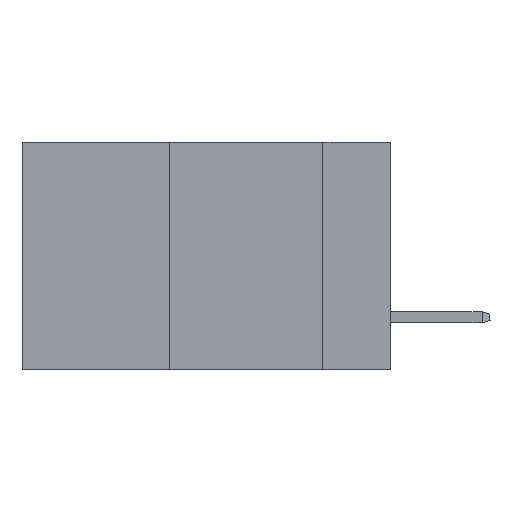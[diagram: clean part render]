
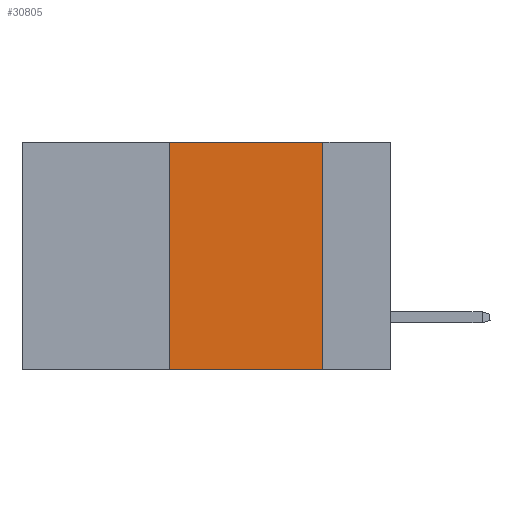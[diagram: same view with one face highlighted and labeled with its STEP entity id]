
A CAD part, left-side view. The second image highlights one B-rep face of the part: STEP entity #30805.
In plain terms, the highlighted planar face has unit normal (-1, 0, 0).
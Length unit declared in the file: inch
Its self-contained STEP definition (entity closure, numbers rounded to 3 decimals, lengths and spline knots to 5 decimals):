
#793 = VERTEX_POINT ( 'NONE', #25462 ) ;
#969 = DIRECTION ( 'NONE',  ( 0., -1., 0. ) ) ;
#1137 = VECTOR ( 'NONE', #1248, 39.37008 ) ;
#1248 = DIRECTION ( 'NONE',  ( 0., -1., 0. ) ) ;
#3968 = VECTOR ( 'NONE', #23589, 39.37008 ) ;
#4035 = CARTESIAN_POINT ( 'NONE',  ( 0., 0.11, 0. ) ) ;
#8801 = EDGE_LOOP ( 'NONE', ( #17705, #30696, #17278, #35074 ) ) ;
#9287 = VERTEX_POINT ( 'NONE', #24749 ) ;
#9835 = CARTESIAN_POINT ( 'NONE',  ( 0., 0.36, 0. ) ) ;
#10026 = VECTOR ( 'NONE', #33247, 39.37008 ) ;
#10438 = LINE ( 'NONE', #22351, #1137 ) ;
#13290 = CARTESIAN_POINT ( 'NONE',  ( 0., 0.6, 0. ) ) ;
#13874 = AXIS2_PLACEMENT_3D ( 'NONE', #13290, #28423, #22605 ) ;
#14196 = EDGE_CURVE ( 'NONE', #793, #27697, #25897, .T. ) ;
#14399 = EDGE_CURVE ( 'NONE', #27697, #33178, #10438, .T. ) ;
#17278 = ORIENTED_EDGE ( 'NONE', *, *, #14196, .F. ) ;
#17705 = ORIENTED_EDGE ( 'NONE', *, *, #26358, .F. ) ;
#19092 = VECTOR ( 'NONE', #969, 39.37008 ) ;
#22351 = CARTESIAN_POINT ( 'NONE',  ( 0., 0.6, 0. ) ) ;
#22605 = DIRECTION ( 'NONE',  ( 0., 0., -1. ) ) ;
#23589 = DIRECTION ( 'NONE',  ( 0., 0., -1. ) ) ;
#24749 = CARTESIAN_POINT ( 'NONE',  ( 0., 0.11, -0.37 ) ) ;
#25462 = CARTESIAN_POINT ( 'NONE',  ( 0., 0.36, -0.37 ) ) ;
#25628 = CARTESIAN_POINT ( 'NONE',  ( 0., 0.36, 0. ) ) ;
#25897 = LINE ( 'NONE', #9835, #10026 ) ;
#26358 = EDGE_CURVE ( 'NONE', #33178, #9287, #38029, .T. ) ;
#26664 = CARTESIAN_POINT ( 'NONE',  ( 0., 0.11, 0. ) ) ;
#27017 = LINE ( 'NONE', #31013, #19092 ) ;
#27697 = VERTEX_POINT ( 'NONE', #25628 ) ;
#28423 = DIRECTION ( 'NONE',  ( 1., 0., 0. ) ) ;
#30696 = ORIENTED_EDGE ( 'NONE', *, *, #14399, .F. ) ;
#30805 = ADVANCED_FACE ( 'NONE', ( #31505 ), #33906, .F. ) ;
#31013 = CARTESIAN_POINT ( 'NONE',  ( 0., 0.6, -0.37 ) ) ;
#31505 = FACE_OUTER_BOUND ( 'NONE', #8801, .T. ) ;
#33178 = VERTEX_POINT ( 'NONE', #4035 ) ;
#33247 = DIRECTION ( 'NONE',  ( 0., 0., 1. ) ) ;
#33906 = PLANE ( 'NONE',  #13874 ) ;
#34040 = EDGE_CURVE ( 'NONE', #793, #9287, #27017, .T. ) ;
#35074 = ORIENTED_EDGE ( 'NONE', *, *, #34040, .T. ) ;
#38029 = LINE ( 'NONE', #26664, #3968 ) ;
